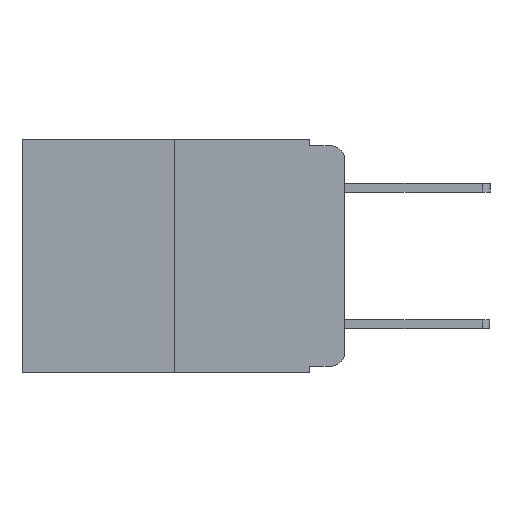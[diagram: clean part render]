
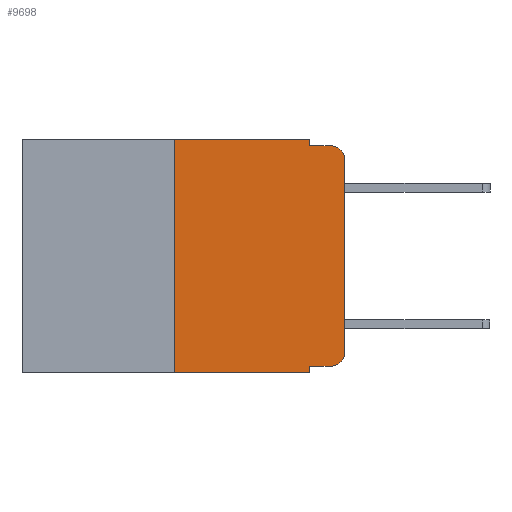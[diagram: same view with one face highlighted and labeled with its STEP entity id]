
A CAD part, left-side view. The second image highlights one B-rep face of the part: STEP entity #9698.
In plain terms, the highlighted planar face has unit normal (-1, 0, 0).
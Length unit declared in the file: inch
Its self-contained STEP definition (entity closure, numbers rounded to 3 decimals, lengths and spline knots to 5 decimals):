
#65 = ORIENTED_EDGE ( 'NONE', *, *, #12988, .F. ) ;
#138 = ORIENTED_EDGE ( 'NONE', *, *, #9708, .F. ) ;
#264 = ORIENTED_EDGE ( 'NONE', *, *, #11961, .F. ) ;
#436 = VERTEX_POINT ( 'NONE', #17138 ) ;
#772 = ORIENTED_EDGE ( 'NONE', *, *, #17043, .T. ) ;
#1087 = VECTOR ( 'NONE', #7094, 39.37008 ) ;
#1091 = ORIENTED_EDGE ( 'NONE', *, *, #10953, .F. ) ;
#1165 = ORIENTED_EDGE ( 'NONE', *, *, #8896, .T. ) ;
#1260 = VERTEX_POINT ( 'NONE', #18420 ) ;
#1321 = ORIENTED_EDGE ( 'NONE', *, *, #7801, .T. ) ;
#1931 = AXIS2_PLACEMENT_3D ( 'NONE', #14440, #5033, #15985 ) ;
#2246 = DIRECTION ( 'NONE',  ( 0., -1., 0. ) ) ;
#2257 = LINE ( 'NONE', #10213, #1087 ) ;
#2260 = CARTESIAN_POINT ( 'NONE',  ( 0., 0., -0.03 ) ) ;
#2803 = PLANE ( 'NONE',  #9874 ) ;
#3156 = VERTEX_POINT ( 'NONE', #5829 ) ;
#3500 = CARTESIAN_POINT ( 'NONE',  ( 0., 0.02, -0.313 ) ) ;
#4735 = CARTESIAN_POINT ( 'NONE',  ( 0., 0.473, -0.343 ) ) ;
#5033 = DIRECTION ( 'NONE',  ( -1., 0., 0. ) ) ;
#5208 = DIRECTION ( 'NONE',  ( 0., 0., -1. ) ) ;
#5829 = CARTESIAN_POINT ( 'NONE',  ( 0., 0.051, -0.01 ) ) ;
#6089 = VERTEX_POINT ( 'NONE', #2260 ) ;
#6253 = DIRECTION ( 'NONE',  ( 0., 0., -1. ) ) ;
#6678 = EDGE_LOOP ( 'NONE', ( #10279, #11041, #11208, #65, #138, #264, #772, #1091, #1165, #1321 ) ) ;
#7094 = DIRECTION ( 'NONE',  ( 0., -1., 0. ) ) ;
#7126 = VERTEX_POINT ( 'NONE', #18825 ) ;
#7661 = DIRECTION ( 'NONE',  ( 0., 0., 1. ) ) ;
#7778 = CARTESIAN_POINT ( 'NONE',  ( 0., 0.051, 0. ) ) ;
#7801 = EDGE_CURVE ( 'NONE', #10333, #10359, #7826, .T. ) ;
#7812 = DIRECTION ( 'NONE',  ( 0., -1., 0. ) ) ;
#7826 = CIRCLE ( 'NONE', #12122, 0.02 ) ;
#8405 = VECTOR ( 'NONE', #7661, 39.37008 ) ;
#8431 = LINE ( 'NONE', #9375, #16159 ) ;
#8896 = EDGE_CURVE ( 'NONE', #16442, #10333, #17272, .T. ) ;
#9375 = CARTESIAN_POINT ( 'NONE',  ( 0., 0., 0. ) ) ;
#9393 = DIRECTION ( 'NONE',  ( 0., 0., -1. ) ) ;
#9511 = LINE ( 'NONE', #20176, #17232 ) ;
#9698 = ADVANCED_FACE ( 'NONE', ( #17731 ), #2803, .F. ) ;
#9708 = EDGE_CURVE ( 'NONE', #1260, #7126, #9511, .T. ) ;
#9874 = AXIS2_PLACEMENT_3D ( 'NONE', #13994, #15540, #6253 ) ;
#10213 = CARTESIAN_POINT ( 'NONE',  ( 0., 0.051, -0.01 ) ) ;
#10279 = ORIENTED_EDGE ( 'NONE', *, *, #18222, .T. ) ;
#10333 = VERTEX_POINT ( 'NONE', #14323 ) ;
#10359 = VERTEX_POINT ( 'NONE', #18998 ) ;
#10416 = VECTOR ( 'NONE', #9393, 39.37008 ) ;
#10756 = CARTESIAN_POINT ( 'NONE',  ( 0., 0.25, 0. ) ) ;
#10911 = DIRECTION ( 'NONE',  ( 0., 0., 1. ) ) ;
#10953 = EDGE_CURVE ( 'NONE', #16442, #436, #20482, .T. ) ;
#11041 = ORIENTED_EDGE ( 'NONE', *, *, #17173, .T. ) ;
#11079 = DIRECTION ( 'NONE',  ( 0., -1., 0. ) ) ;
#11113 = CIRCLE ( 'NONE', #1931, 0.02 ) ;
#11208 = ORIENTED_EDGE ( 'NONE', *, *, #16113, .F. ) ;
#11247 = CARTESIAN_POINT ( 'NONE',  ( 0., 0.02, -0.01 ) ) ;
#11961 = EDGE_CURVE ( 'NONE', #19341, #1260, #16614, .T. ) ;
#12122 = AXIS2_PLACEMENT_3D ( 'NONE', #3500, #14586, #5208 ) ;
#12988 = EDGE_CURVE ( 'NONE', #7126, #3156, #19479, .T. ) ;
#13518 = VECTOR ( 'NONE', #11079, 39.37008 ) ;
#13994 = CARTESIAN_POINT ( 'NONE',  ( 0., 0.473, 0. ) ) ;
#14202 = CARTESIAN_POINT ( 'NONE',  ( 0., 0.051, -0.333 ) ) ;
#14323 = CARTESIAN_POINT ( 'NONE',  ( 0., 0.02, -0.333 ) ) ;
#14440 = CARTESIAN_POINT ( 'NONE',  ( 0., 0.02, -0.03 ) ) ;
#14586 = DIRECTION ( 'NONE',  ( -1., 0., 0. ) ) ;
#15083 = CARTESIAN_POINT ( 'NONE',  ( 0., 0.051, -0.333 ) ) ;
#15360 = VECTOR ( 'NONE', #16302, 39.37008 ) ;
#15540 = DIRECTION ( 'NONE',  ( 1., 0., 0. ) ) ;
#15985 = DIRECTION ( 'NONE',  ( 0., 0., -1. ) ) ;
#16113 = EDGE_CURVE ( 'NONE', #3156, #19652, #2257, .T. ) ;
#16159 = VECTOR ( 'NONE', #10911, 39.37008 ) ;
#16302 = DIRECTION ( 'NONE',  ( 0., 0., -1. ) ) ;
#16442 = VERTEX_POINT ( 'NONE', #14202 ) ;
#16614 = LINE ( 'NONE', #10756, #8405 ) ;
#17043 = EDGE_CURVE ( 'NONE', #19341, #436, #17169, .T. ) ;
#17138 = CARTESIAN_POINT ( 'NONE',  ( 0., 0.051, -0.343 ) ) ;
#17169 = LINE ( 'NONE', #4735, #13518 ) ;
#17173 = EDGE_CURVE ( 'NONE', #6089, #19652, #11113, .T. ) ;
#17232 = VECTOR ( 'NONE', #7812, 39.37008 ) ;
#17272 = LINE ( 'NONE', #15083, #20345 ) ;
#17731 = FACE_OUTER_BOUND ( 'NONE', #6678, .T. ) ;
#17832 = CARTESIAN_POINT ( 'NONE',  ( 0., 0.051, 0. ) ) ;
#18178 = CARTESIAN_POINT ( 'NONE',  ( 0., 0.25, -0.343 ) ) ;
#18222 = EDGE_CURVE ( 'NONE', #10359, #6089, #8431, .T. ) ;
#18420 = CARTESIAN_POINT ( 'NONE',  ( 0., 0.25, 0. ) ) ;
#18825 = CARTESIAN_POINT ( 'NONE',  ( 0., 0.051, 0. ) ) ;
#18998 = CARTESIAN_POINT ( 'NONE',  ( 0., 0., -0.313 ) ) ;
#19341 = VERTEX_POINT ( 'NONE', #18178 ) ;
#19479 = LINE ( 'NONE', #17832, #15360 ) ;
#19652 = VERTEX_POINT ( 'NONE', #11247 ) ;
#20176 = CARTESIAN_POINT ( 'NONE',  ( 0., 0.473, 0. ) ) ;
#20345 = VECTOR ( 'NONE', #2246, 39.37008 ) ;
#20482 = LINE ( 'NONE', #7778, #10416 ) ;
